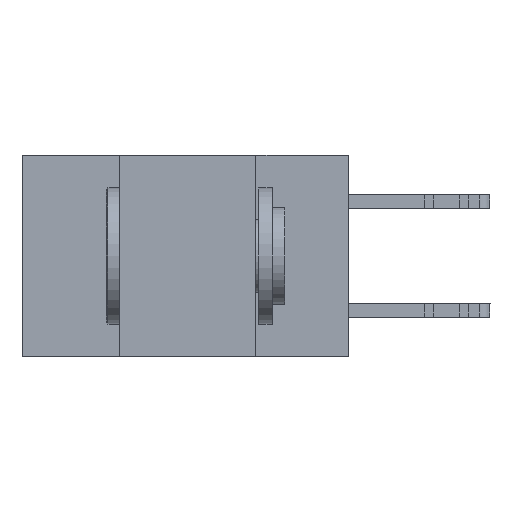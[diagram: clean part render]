
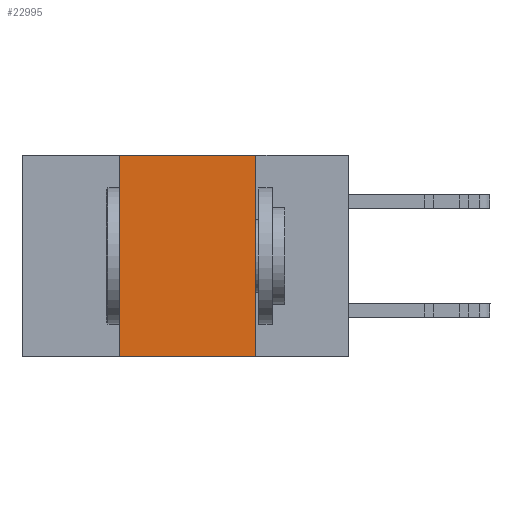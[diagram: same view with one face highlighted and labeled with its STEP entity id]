
A CAD part, left-side view. The second image highlights one B-rep face of the part: STEP entity #22995.
In plain terms, the highlighted planar face has unit normal (-1, 0, 0).
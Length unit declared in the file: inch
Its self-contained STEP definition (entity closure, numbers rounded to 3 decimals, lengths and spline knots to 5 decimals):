
#1541 = DIRECTION ( 'NONE',  ( 0., 0., 1. ) ) ;
#3494 = LINE ( 'NONE', #6943, #18015 ) ;
#3503 = VERTEX_POINT ( 'NONE', #25343 ) ;
#5361 = DIRECTION ( 'NONE',  ( 0., -1., 0. ) ) ;
#6943 = CARTESIAN_POINT ( 'NONE',  ( 0., 0.42, 0. ) ) ;
#6978 = AXIS2_PLACEMENT_3D ( 'NONE', #21995, #27166, #29882 ) ;
#8212 = VECTOR ( 'NONE', #5361, 39.37008 ) ;
#10057 = VERTEX_POINT ( 'NONE', #19470 ) ;
#10268 = EDGE_CURVE ( 'NONE', #3503, #31539, #31289, .T. ) ;
#11895 = PLANE ( 'NONE',  #6978 ) ;
#12399 = DIRECTION ( 'NONE',  ( 0., -1., 0. ) ) ;
#13233 = CARTESIAN_POINT ( 'NONE',  ( 0., 0.42, -0.37 ) ) ;
#14003 = VECTOR ( 'NONE', #27768, 39.37008 ) ;
#17595 = CARTESIAN_POINT ( 'NONE',  ( 0., 0.6, 0. ) ) ;
#17819 = EDGE_CURVE ( 'NONE', #24259, #10057, #3494, .T. ) ;
#18015 = VECTOR ( 'NONE', #1541, 39.37008 ) ;
#18130 = FACE_OUTER_BOUND ( 'NONE', #22009, .T. ) ;
#19470 = CARTESIAN_POINT ( 'NONE',  ( 0., 0.42, 0. ) ) ;
#20258 = ORIENTED_EDGE ( 'NONE', *, *, #10268, .F. ) ;
#21995 = CARTESIAN_POINT ( 'NONE',  ( 0., 0.6, 0. ) ) ;
#22009 = EDGE_LOOP ( 'NONE', ( #20258, #25166, #24176, #30186 ) ) ;
#22117 = LINE ( 'NONE', #17595, #29335 ) ;
#22519 = CARTESIAN_POINT ( 'NONE',  ( 0., 0.17, -0.37 ) ) ;
#22995 = ADVANCED_FACE ( 'NONE', ( #18130 ), #11895, .F. ) ;
#24176 = ORIENTED_EDGE ( 'NONE', *, *, #17819, .F. ) ;
#24259 = VERTEX_POINT ( 'NONE', #13233 ) ;
#25166 = ORIENTED_EDGE ( 'NONE', *, *, #29534, .F. ) ;
#25186 = CARTESIAN_POINT ( 'NONE',  ( 0., 0.17, 0. ) ) ;
#25343 = CARTESIAN_POINT ( 'NONE',  ( 0., 0.17, 0. ) ) ;
#25940 = LINE ( 'NONE', #33266, #8212 ) ;
#26059 = EDGE_CURVE ( 'NONE', #24259, #31539, #25940, .T. ) ;
#27166 = DIRECTION ( 'NONE',  ( 1., 0., 0. ) ) ;
#27768 = DIRECTION ( 'NONE',  ( 0., 0., -1. ) ) ;
#29335 = VECTOR ( 'NONE', #12399, 39.37008 ) ;
#29534 = EDGE_CURVE ( 'NONE', #10057, #3503, #22117, .T. ) ;
#29882 = DIRECTION ( 'NONE',  ( 0., 0., -1. ) ) ;
#30186 = ORIENTED_EDGE ( 'NONE', *, *, #26059, .T. ) ;
#31289 = LINE ( 'NONE', #25186, #14003 ) ;
#31539 = VERTEX_POINT ( 'NONE', #22519 ) ;
#33266 = CARTESIAN_POINT ( 'NONE',  ( 0., 0.6, -0.37 ) ) ;
